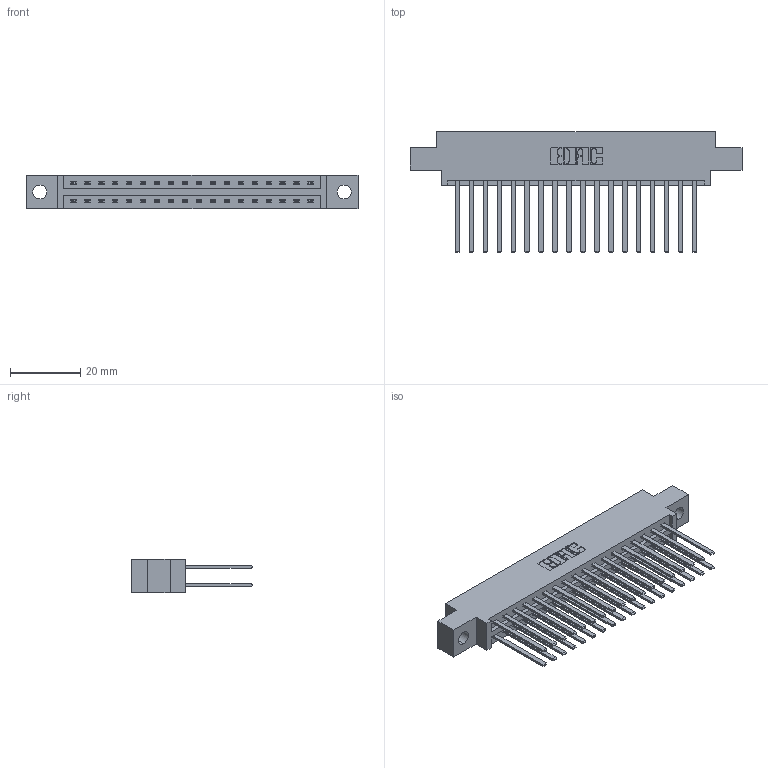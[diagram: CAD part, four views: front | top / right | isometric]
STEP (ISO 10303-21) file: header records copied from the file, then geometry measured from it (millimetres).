
FILE_DESCRIPTION (( 'STEP AP203' ), '1' );
FILE_NAME ('387-036-544-804.STEP', '2019-10-17T19:45:38', ( '' ), ( '' ), 'SwSTEP 2.0', 'SolidWorks 2016', '' );
FILE_SCHEMA (( 'CONFIG_CONTROL_DESIGN' ));
Length unit declared in the file: inch
Products named in the file (3): 345-292-001_345-293-144; 387-036-544-804; 337 Part_0.170 Offset - 0.156 Dia-TH
Assembly tree (37 placements, depth 2):
  387-036-544-804
    337 Part_0.170 Offset - 0.156 Dia-TH
    345-292-001_345-293-144  x36
Bounding box: 94.34 x 34.3 x 9.4 mm (x, y, z)
Volume: 9921.7 mm3; surface area: 12537.1 mm2
Topology: 37 solids, 37 shells, 1846 faces, 5471 edges, 3598 vertices
Faces by surface type: plane 1298, cylinder 548
Entity records: 17011 total; most frequent: CARTESIAN_POINT 2886, ORIENTED_EDGE 2822, DIRECTION 2495, EDGE_CURVE 1411, LINE 1287, VECTOR 1287, VERTEX_POINT 938, AXIS2_PLACEMENT_3D 604
